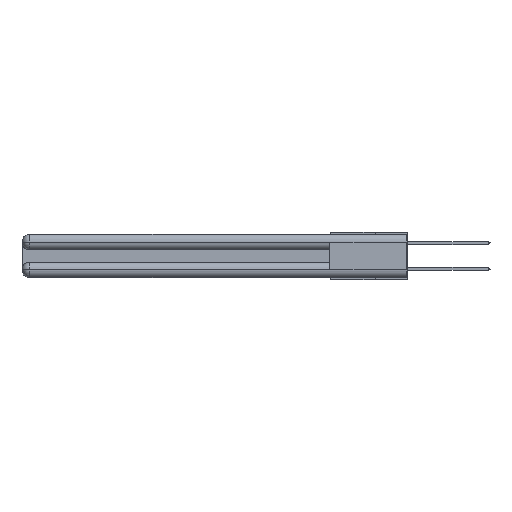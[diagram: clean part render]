
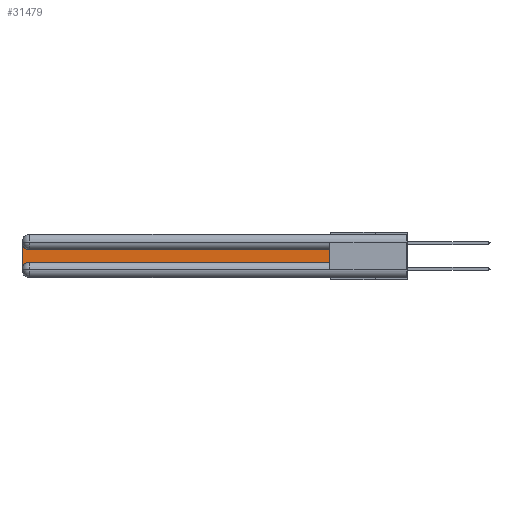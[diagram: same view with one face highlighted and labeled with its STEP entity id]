
A CAD part, left-side view. The second image highlights one B-rep face of the part: STEP entity #31479.
In plain terms, the highlighted planar face has unit normal (-1, 0, 0).
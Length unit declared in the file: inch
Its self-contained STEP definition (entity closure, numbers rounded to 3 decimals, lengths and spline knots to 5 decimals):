
#29 = EDGE_CURVE ( 'NONE', #30094, #31950, #22575, .T. ) ;
#40 = DIRECTION ( 'NONE',  ( 0., 0., -1. ) ) ;
#961 = ORIENTED_EDGE ( 'NONE', *, *, #29, .T. ) ;
#1570 = VERTEX_POINT ( 'NONE', #15698 ) ;
#3258 = DIRECTION ( 'NONE',  ( 0., 0., -1. ) ) ;
#3856 = LINE ( 'NONE', #8227, #31576 ) ;
#4119 = CARTESIAN_POINT ( 'NONE',  ( 0.075, 3., -0.1225 ) ) ;
#4281 = DIRECTION ( 'NONE',  ( 0., -1., 0. ) ) ;
#4877 = CARTESIAN_POINT ( 'NONE',  ( 0.075, 0.6, -0.2175 ) ) ;
#5059 = DIRECTION ( 'NONE',  ( 1., 0., 0. ) ) ;
#6234 = CIRCLE ( 'NONE', #18790, 0.06 ) ;
#7227 = CARTESIAN_POINT ( 'NONE',  ( 0.075, 3., -0.2775 ) ) ;
#7847 = CIRCLE ( 'NONE', #18019, 0.06 ) ;
#8227 = CARTESIAN_POINT ( 'NONE',  ( 0.075, 3., -0.2175 ) ) ;
#10274 = VERTEX_POINT ( 'NONE', #7227 ) ;
#10505 = ORIENTED_EDGE ( 'NONE', *, *, #17867, .T. ) ;
#10540 = ORIENTED_EDGE ( 'NONE', *, *, #19458, .T. ) ;
#10834 = LINE ( 'NONE', #27351, #26519 ) ;
#11397 = CARTESIAN_POINT ( 'NONE',  ( 0.075, 0.6, -0.1225 ) ) ;
#11507 = DIRECTION ( 'NONE',  ( 1., 0., 0. ) ) ;
#11550 = EDGE_LOOP ( 'NONE', ( #22553, #15452, #10540, #32237, #10505, #961 ) ) ;
#11649 = AXIS2_PLACEMENT_3D ( 'NONE', #4119, #16720, #11674 ) ;
#11674 = DIRECTION ( 'NONE',  ( 0., 0., -1. ) ) ;
#11912 = EDGE_CURVE ( 'NONE', #10274, #1570, #7847, .T. ) ;
#12744 = DIRECTION ( 'NONE',  ( 0., 0., 1. ) ) ;
#15452 = ORIENTED_EDGE ( 'NONE', *, *, #20770, .T. ) ;
#15698 = CARTESIAN_POINT ( 'NONE',  ( 0.075, 2.94, -0.2175 ) ) ;
#16720 = DIRECTION ( 'NONE',  ( 1., 0., 0. ) ) ;
#16792 = CARTESIAN_POINT ( 'NONE',  ( 0.075, 3., -0.0625 ) ) ;
#17867 = EDGE_CURVE ( 'NONE', #1570, #30094, #10834, .T. ) ;
#18019 = AXIS2_PLACEMENT_3D ( 'NONE', #28602, #11507, #24302 ) ;
#18790 = AXIS2_PLACEMENT_3D ( 'NONE', #23124, #5059, #40 ) ;
#19116 = VECTOR ( 'NONE', #24953, 39.37008 ) ;
#19458 = EDGE_CURVE ( 'NONE', #26500, #10274, #3856, .T. ) ;
#20770 = EDGE_CURVE ( 'NONE', #30395, #26500, #6234, .T. ) ;
#22553 = ORIENTED_EDGE ( 'NONE', *, *, #27724, .T. ) ;
#22575 = LINE ( 'NONE', #4877, #25395 ) ;
#23124 = CARTESIAN_POINT ( 'NONE',  ( 0.075, 2.94, -0.0625 ) ) ;
#24302 = DIRECTION ( 'NONE',  ( 0., 0., -1. ) ) ;
#24953 = DIRECTION ( 'NONE',  ( 0., 1., 0. ) ) ;
#25395 = VECTOR ( 'NONE', #12744, 39.37008 ) ;
#26500 = VERTEX_POINT ( 'NONE', #16792 ) ;
#26519 = VECTOR ( 'NONE', #4281, 39.37008 ) ;
#26728 = LINE ( 'NONE', #30028, #19116 ) ;
#27320 = CARTESIAN_POINT ( 'NONE',  ( 0.075, 0.6, -0.2175 ) ) ;
#27351 = CARTESIAN_POINT ( 'NONE',  ( 0.075, 0.6, -0.2175 ) ) ;
#27724 = EDGE_CURVE ( 'NONE', #31950, #30395, #26728, .T. ) ;
#28602 = CARTESIAN_POINT ( 'NONE',  ( 0.075, 2.94, -0.2775 ) ) ;
#30028 = CARTESIAN_POINT ( 'NONE',  ( 0.075, 0.6, -0.1225 ) ) ;
#30094 = VERTEX_POINT ( 'NONE', #27320 ) ;
#30395 = VERTEX_POINT ( 'NONE', #32203 ) ;
#31479 = ADVANCED_FACE ( 'NONE', ( #32094 ), #31863, .F. ) ;
#31576 = VECTOR ( 'NONE', #3258, 39.37008 ) ;
#31863 = PLANE ( 'NONE',  #11649 ) ;
#31950 = VERTEX_POINT ( 'NONE', #11397 ) ;
#32094 = FACE_OUTER_BOUND ( 'NONE', #11550, .T. ) ;
#32203 = CARTESIAN_POINT ( 'NONE',  ( 0.075, 2.94, -0.1225 ) ) ;
#32237 = ORIENTED_EDGE ( 'NONE', *, *, #11912, .T. ) ;
